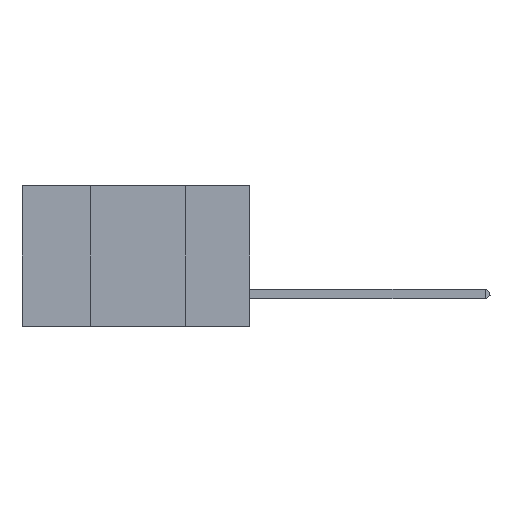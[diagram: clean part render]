
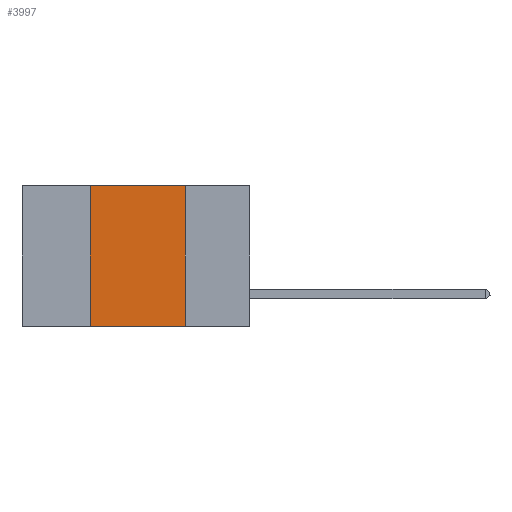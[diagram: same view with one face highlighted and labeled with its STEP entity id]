
A CAD part, left-side view. The second image highlights one B-rep face of the part: STEP entity #3997.
In plain terms, the highlighted planar face has unit normal (-1, 0, 0).
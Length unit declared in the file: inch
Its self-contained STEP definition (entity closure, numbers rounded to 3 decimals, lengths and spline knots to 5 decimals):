
#274 = CARTESIAN_POINT ( 'NONE',  ( 0., 0.6, -0.37 ) ) ;
#394 = LINE ( 'NONE', #274, #11599 ) ;
#893 = EDGE_CURVE ( 'NONE', #15326, #18844, #11806, .T. ) ;
#1569 = ORIENTED_EDGE ( 'NONE', *, *, #893, .F. ) ;
#3185 = DIRECTION ( 'NONE',  ( 0., 0., 1. ) ) ;
#3997 = ADVANCED_FACE ( 'NONE', ( #21347 ), #11816, .F. ) ;
#4429 = CARTESIAN_POINT ( 'NONE',  ( 0., 0.17, -0.37 ) ) ;
#4520 = EDGE_LOOP ( 'NONE', ( #16241, #5431, #1569, #9041 ) ) ;
#5390 = EDGE_CURVE ( 'NONE', #15326, #18459, #394, .T. ) ;
#5431 = ORIENTED_EDGE ( 'NONE', *, *, #14796, .F. ) ;
#5682 = EDGE_CURVE ( 'NONE', #19656, #18459, #8953, .T. ) ;
#5982 = DIRECTION ( 'NONE',  ( 1., 0., 0. ) ) ;
#6893 = VECTOR ( 'NONE', #3185, 39.37008 ) ;
#7341 = CARTESIAN_POINT ( 'NONE',  ( 0., 0.42, 0. ) ) ;
#7831 = DIRECTION ( 'NONE',  ( 0., 0., -1. ) ) ;
#8693 = CARTESIAN_POINT ( 'NONE',  ( 0., 0.42, -0.37 ) ) ;
#8953 = LINE ( 'NONE', #19039, #17573 ) ;
#9041 = ORIENTED_EDGE ( 'NONE', *, *, #5390, .T. ) ;
#10349 = DIRECTION ( 'NONE',  ( 0., -1., 0. ) ) ;
#11423 = DIRECTION ( 'NONE',  ( 0., -1., 0. ) ) ;
#11599 = VECTOR ( 'NONE', #11423, 39.37008 ) ;
#11806 = LINE ( 'NONE', #23394, #6893 ) ;
#11816 = PLANE ( 'NONE',  #21687 ) ;
#13129 = VECTOR ( 'NONE', #10349, 39.37008 ) ;
#13635 = CARTESIAN_POINT ( 'NONE',  ( 0., 0.6, 0. ) ) ;
#14796 = EDGE_CURVE ( 'NONE', #18844, #19656, #16527, .T. ) ;
#15326 = VERTEX_POINT ( 'NONE', #8693 ) ;
#16241 = ORIENTED_EDGE ( 'NONE', *, *, #5682, .F. ) ;
#16527 = LINE ( 'NONE', #19222, #13129 ) ;
#17573 = VECTOR ( 'NONE', #20698, 39.37008 ) ;
#18238 = CARTESIAN_POINT ( 'NONE',  ( 0., 0.17, 0. ) ) ;
#18459 = VERTEX_POINT ( 'NONE', #4429 ) ;
#18844 = VERTEX_POINT ( 'NONE', #7341 ) ;
#19039 = CARTESIAN_POINT ( 'NONE',  ( 0., 0.17, 0. ) ) ;
#19222 = CARTESIAN_POINT ( 'NONE',  ( 0., 0.6, 0. ) ) ;
#19656 = VERTEX_POINT ( 'NONE', #18238 ) ;
#20698 = DIRECTION ( 'NONE',  ( 0., 0., -1. ) ) ;
#21347 = FACE_OUTER_BOUND ( 'NONE', #4520, .T. ) ;
#21687 = AXIS2_PLACEMENT_3D ( 'NONE', #13635, #5982, #7831 ) ;
#23394 = CARTESIAN_POINT ( 'NONE',  ( 0., 0.42, 0. ) ) ;
